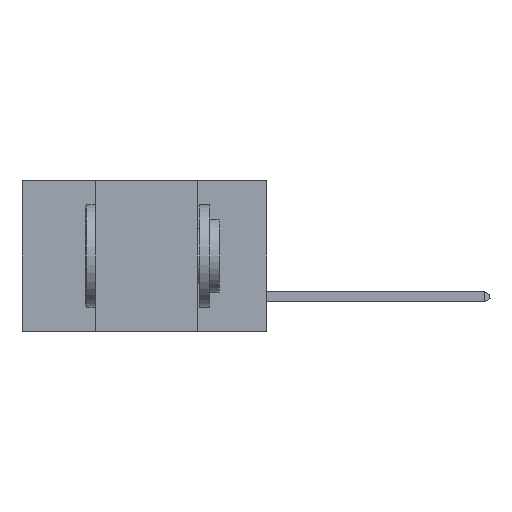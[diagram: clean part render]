
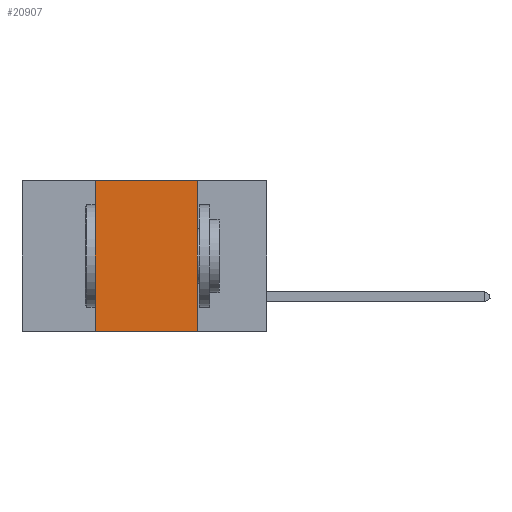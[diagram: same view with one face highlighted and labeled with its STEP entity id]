
A CAD part, left-side view. The second image highlights one B-rep face of the part: STEP entity #20907.
In plain terms, the highlighted planar face has unit normal (-1, 0, 0).
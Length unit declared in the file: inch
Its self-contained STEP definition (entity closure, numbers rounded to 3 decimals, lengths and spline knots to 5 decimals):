
#212 = CARTESIAN_POINT ( 'NONE',  ( 0., 0.42, 0. ) ) ;
#1172 = LINE ( 'NONE', #7317, #20591 ) ;
#1716 = CARTESIAN_POINT ( 'NONE',  ( 0., 0.17, 0. ) ) ;
#2190 = CARTESIAN_POINT ( 'NONE',  ( 0., 0.17, 0. ) ) ;
#2204 = VERTEX_POINT ( 'NONE', #212 ) ;
#3151 = EDGE_CURVE ( 'NONE', #2204, #16084, #15554, .T. ) ;
#3795 = LINE ( 'NONE', #1716, #29568 ) ;
#4349 = EDGE_LOOP ( 'NONE', ( #18281, #13263, #25215, #18310 ) ) ;
#6264 = DIRECTION ( 'NONE',  ( 1., 0., 0. ) ) ;
#7317 = CARTESIAN_POINT ( 'NONE',  ( 0., 0.6, -0.37 ) ) ;
#8736 = EDGE_CURVE ( 'NONE', #16084, #18939, #3795, .T. ) ;
#10431 = FACE_OUTER_BOUND ( 'NONE', #4349, .T. ) ;
#10676 = AXIS2_PLACEMENT_3D ( 'NONE', #16326, #6264, #23766 ) ;
#13263 = ORIENTED_EDGE ( 'NONE', *, *, #3151, .F. ) ;
#14803 = CARTESIAN_POINT ( 'NONE',  ( 0., 0.42, -0.37 ) ) ;
#15554 = LINE ( 'NONE', #25792, #22892 ) ;
#16084 = VERTEX_POINT ( 'NONE', #2190 ) ;
#16326 = CARTESIAN_POINT ( 'NONE',  ( 0., 0.6, 0. ) ) ;
#17138 = LINE ( 'NONE', #32125, #23697 ) ;
#18164 = CARTESIAN_POINT ( 'NONE',  ( 0., 0.17, -0.37 ) ) ;
#18281 = ORIENTED_EDGE ( 'NONE', *, *, #8736, .F. ) ;
#18310 = ORIENTED_EDGE ( 'NONE', *, *, #20565, .T. ) ;
#18939 = VERTEX_POINT ( 'NONE', #18164 ) ;
#20565 = EDGE_CURVE ( 'NONE', #21139, #18939, #1172, .T. ) ;
#20591 = VECTOR ( 'NONE', #32237, 39.37008 ) ;
#20907 = ADVANCED_FACE ( 'NONE', ( #10431 ), #23651, .F. ) ;
#21139 = VERTEX_POINT ( 'NONE', #14803 ) ;
#22892 = VECTOR ( 'NONE', #25832, 39.37008 ) ;
#23651 = PLANE ( 'NONE',  #10676 ) ;
#23697 = VECTOR ( 'NONE', #27291, 39.37008 ) ;
#23766 = DIRECTION ( 'NONE',  ( 0., 0., -1. ) ) ;
#25215 = ORIENTED_EDGE ( 'NONE', *, *, #25971, .F. ) ;
#25792 = CARTESIAN_POINT ( 'NONE',  ( 0., 0.6, 0. ) ) ;
#25832 = DIRECTION ( 'NONE',  ( 0., -1., 0. ) ) ;
#25971 = EDGE_CURVE ( 'NONE', #21139, #2204, #17138, .T. ) ;
#26826 = DIRECTION ( 'NONE',  ( 0., 0., -1. ) ) ;
#27291 = DIRECTION ( 'NONE',  ( 0., 0., 1. ) ) ;
#29568 = VECTOR ( 'NONE', #26826, 39.37008 ) ;
#32125 = CARTESIAN_POINT ( 'NONE',  ( 0., 0.42, 0. ) ) ;
#32237 = DIRECTION ( 'NONE',  ( 0., -1., 0. ) ) ;
